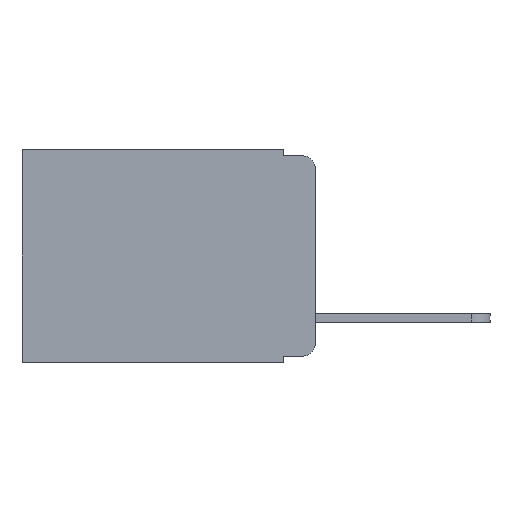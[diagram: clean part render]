
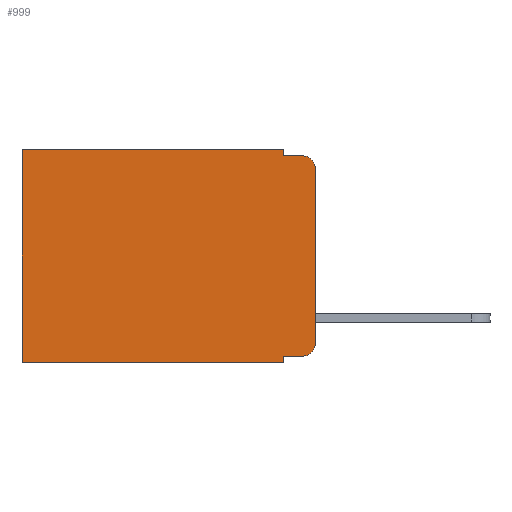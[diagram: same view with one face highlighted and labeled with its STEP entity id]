
A CAD part, left-side view. The second image highlights one B-rep face of the part: STEP entity #999.
In plain terms, the highlighted planar face has unit normal (-1, 0, 0).
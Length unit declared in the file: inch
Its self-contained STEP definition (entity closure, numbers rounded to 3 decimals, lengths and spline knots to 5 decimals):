
#56 = DIRECTION ( 'NONE',  ( 1., 0., 0. ) ) ;
#239 = VECTOR ( 'NONE', #1271, 39.37008 ) ;
#289 = EDGE_CURVE ( 'NONE', #7349, #6124, #1607, .T. ) ;
#477 = DIRECTION ( 'NONE',  ( 0., 0., -1. ) ) ;
#567 = VECTOR ( 'NONE', #7235, 39.37008 ) ;
#611 = LINE ( 'NONE', #1970, #4689 ) ;
#666 = VERTEX_POINT ( 'NONE', #8266 ) ;
#757 = EDGE_CURVE ( 'NONE', #7349, #6465, #4682, .T. ) ;
#763 = ORIENTED_EDGE ( 'NONE', *, *, #8981, .F. ) ;
#802 = CARTESIAN_POINT ( 'NONE',  ( 0.298, 0.051, 0. ) ) ;
#861 = CARTESIAN_POINT ( 'NONE',  ( 0.298, 0.473, 0. ) ) ;
#999 = ADVANCED_FACE ( 'NONE', ( #9688 ), #4892, .F. ) ;
#1010 = VERTEX_POINT ( 'NONE', #4202 ) ;
#1115 = CARTESIAN_POINT ( 'NONE',  ( 0.298, 0.051, -0.333 ) ) ;
#1271 = DIRECTION ( 'NONE',  ( 0., -1., 0. ) ) ;
#1325 = CARTESIAN_POINT ( 'NONE',  ( 0.298, 0., 0. ) ) ;
#1345 = CIRCLE ( 'NONE', #7868, 0.02 ) ;
#1407 = DIRECTION ( 'NONE',  ( 0., -1., 0. ) ) ;
#1416 = CARTESIAN_POINT ( 'NONE',  ( 0.298, 0., -0.343 ) ) ;
#1444 = CARTESIAN_POINT ( 'NONE',  ( 0.298, 0.051, -0.01 ) ) ;
#1482 = CARTESIAN_POINT ( 'NONE',  ( 0.298, 0.051, -0.01 ) ) ;
#1544 = CIRCLE ( 'NONE', #3111, 0.02 ) ;
#1607 = LINE ( 'NONE', #1115, #2235 ) ;
#1702 = VECTOR ( 'NONE', #477, 39.37008 ) ;
#1747 = DIRECTION ( 'NONE',  ( 0., 1., 0. ) ) ;
#1794 = ORIENTED_EDGE ( 'NONE', *, *, #6660, .F. ) ;
#1970 = CARTESIAN_POINT ( 'NONE',  ( 0.298, 0., 0. ) ) ;
#2023 = ORIENTED_EDGE ( 'NONE', *, *, #7637, .T. ) ;
#2037 = ORIENTED_EDGE ( 'NONE', *, *, #2630, .F. ) ;
#2153 = DIRECTION ( 'NONE',  ( 0., 0., -1. ) ) ;
#2174 = CARTESIAN_POINT ( 'NONE',  ( 0.298, 0.051, -0.333 ) ) ;
#2235 = VECTOR ( 'NONE', #1407, 39.37008 ) ;
#2391 = EDGE_CURVE ( 'NONE', #6465, #3591, #2931, .T. ) ;
#2495 = LINE ( 'NONE', #2878, #6128 ) ;
#2530 = VECTOR ( 'NONE', #5431, 39.37008 ) ;
#2630 = EDGE_CURVE ( 'NONE', #8384, #666, #611, .T. ) ;
#2721 = DIRECTION ( 'NONE',  ( 0., 0., -1. ) ) ;
#2782 = CARTESIAN_POINT ( 'NONE',  ( 0.298, 0.02, -0.333 ) ) ;
#2799 = ORIENTED_EDGE ( 'NONE', *, *, #7095, .T. ) ;
#2878 = CARTESIAN_POINT ( 'NONE',  ( 0.298, 0., 0. ) ) ;
#2931 = LINE ( 'NONE', #1416, #5064 ) ;
#3111 = AXIS2_PLACEMENT_3D ( 'NONE', #3821, #9373, #9168 ) ;
#3411 = CARTESIAN_POINT ( 'NONE',  ( 0.298, 0.051, -0.343 ) ) ;
#3461 = AXIS2_PLACEMENT_3D ( 'NONE', #1325, #56, #9196 ) ;
#3591 = VERTEX_POINT ( 'NONE', #8343 ) ;
#3811 = DIRECTION ( 'NONE',  ( 0., 1., 0. ) ) ;
#3821 = CARTESIAN_POINT ( 'NONE',  ( 0.298, 0.02, -0.313 ) ) ;
#4013 = EDGE_CURVE ( 'NONE', #1010, #3591, #4651, .T. ) ;
#4134 = EDGE_LOOP ( 'NONE', ( #2037, #2023, #1794, #763, #2799, #7129, #5656, #5426, #5221, #5279 ) ) ;
#4201 = EDGE_CURVE ( 'NONE', #6124, #666, #1544, .T. ) ;
#4202 = CARTESIAN_POINT ( 'NONE',  ( 0.298, 0.473, 0. ) ) ;
#4577 = CARTESIAN_POINT ( 'NONE',  ( 0.298, 0.02, -0.01 ) ) ;
#4651 = LINE ( 'NONE', #861, #567 ) ;
#4678 = CARTESIAN_POINT ( 'NONE',  ( 0.298, 0.051, 0. ) ) ;
#4682 = LINE ( 'NONE', #802, #1702 ) ;
#4689 = VECTOR ( 'NONE', #2721, 39.37008 ) ;
#4892 = PLANE ( 'NONE',  #3461 ) ;
#5064 = VECTOR ( 'NONE', #3811, 39.37008 ) ;
#5204 = CARTESIAN_POINT ( 'NONE',  ( 0.298, 0.02, -0.03 ) ) ;
#5221 = ORIENTED_EDGE ( 'NONE', *, *, #289, .T. ) ;
#5279 = ORIENTED_EDGE ( 'NONE', *, *, #4201, .T. ) ;
#5426 = ORIENTED_EDGE ( 'NONE', *, *, #757, .F. ) ;
#5431 = DIRECTION ( 'NONE',  ( 0., 0., -1. ) ) ;
#5514 = VERTEX_POINT ( 'NONE', #4577 ) ;
#5656 = ORIENTED_EDGE ( 'NONE', *, *, #2391, .F. ) ;
#5964 = VERTEX_POINT ( 'NONE', #8380 ) ;
#6124 = VERTEX_POINT ( 'NONE', #2782 ) ;
#6128 = VECTOR ( 'NONE', #1747, 39.37008 ) ;
#6465 = VERTEX_POINT ( 'NONE', #3411 ) ;
#6660 = EDGE_CURVE ( 'NONE', #8489, #5514, #8182, .T. ) ;
#7095 = EDGE_CURVE ( 'NONE', #5964, #1010, #2495, .T. ) ;
#7129 = ORIENTED_EDGE ( 'NONE', *, *, #4013, .T. ) ;
#7235 = DIRECTION ( 'NONE',  ( 0., 0., -1. ) ) ;
#7349 = VERTEX_POINT ( 'NONE', #2174 ) ;
#7637 = EDGE_CURVE ( 'NONE', #8384, #5514, #1345, .T. ) ;
#7868 = AXIS2_PLACEMENT_3D ( 'NONE', #5204, #8495, #2153 ) ;
#8182 = LINE ( 'NONE', #1444, #239 ) ;
#8266 = CARTESIAN_POINT ( 'NONE',  ( 0.298, 0., -0.313 ) ) ;
#8293 = CARTESIAN_POINT ( 'NONE',  ( 0.298, 0., -0.03 ) ) ;
#8343 = CARTESIAN_POINT ( 'NONE',  ( 0.298, 0.473, -0.343 ) ) ;
#8380 = CARTESIAN_POINT ( 'NONE',  ( 0.298, 0.051, 0. ) ) ;
#8384 = VERTEX_POINT ( 'NONE', #8293 ) ;
#8409 = LINE ( 'NONE', #4678, #2530 ) ;
#8489 = VERTEX_POINT ( 'NONE', #1482 ) ;
#8495 = DIRECTION ( 'NONE',  ( -1., 0., 0. ) ) ;
#8981 = EDGE_CURVE ( 'NONE', #5964, #8489, #8409, .T. ) ;
#9168 = DIRECTION ( 'NONE',  ( 0., 0., -1. ) ) ;
#9196 = DIRECTION ( 'NONE',  ( 0., 0., -1. ) ) ;
#9373 = DIRECTION ( 'NONE',  ( -1., 0., 0. ) ) ;
#9688 = FACE_OUTER_BOUND ( 'NONE', #4134, .T. ) ;
